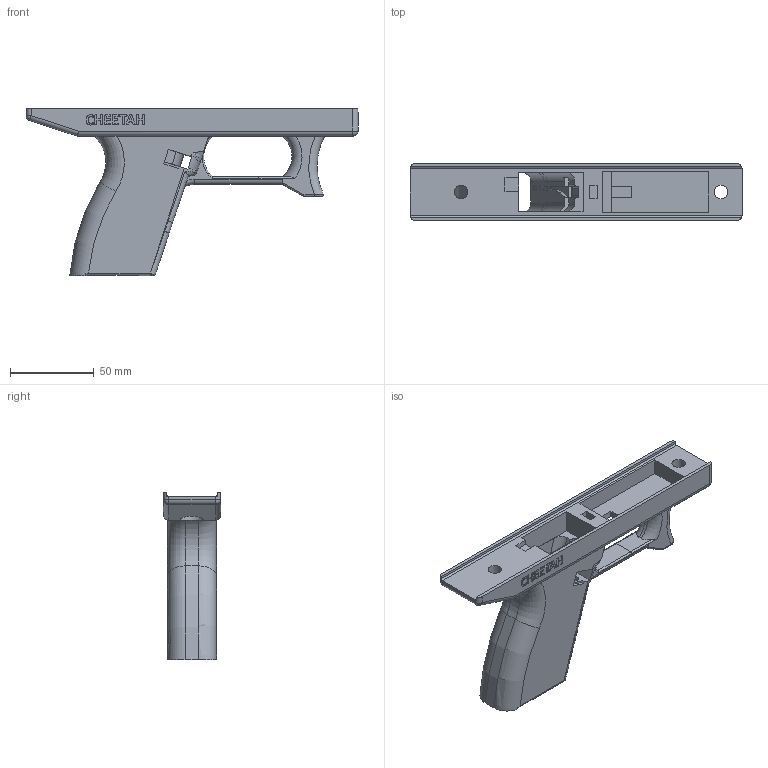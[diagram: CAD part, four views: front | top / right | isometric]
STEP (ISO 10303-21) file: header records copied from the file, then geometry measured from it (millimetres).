
FILE_DESCRIPTION(/* description */ (''),/* implementation_level */ '2;1');
FILE_NAME(/* name */ '',/* time_stamp */ '',/* author */ (''),/* organization */ (''),/* preprocessor_version */ 'ST-DEVELOPER v18.1',/* originating_system */ 'Autodesk Translation Framework v9.7.1.1290',/* authorisation */ '');
FILE_SCHEMA (('AUTOMOTIVE_DESIGN { 1 0 10303 214 3 1 1 }'));
Length unit declared in the file: millimetre
Products named in the file (1): Lower Receiver Body
Bounding box: 198 x 34 x 99.64 mm (x, y, z)
Volume: 126286.1 mm3; surface area: 50948.4 mm2
Topology: 1 solids, 2 shells, 562 faces, 1615 edges, 1061 vertices
Faces by surface type: bspline 256, plane 197, cylinder 82, torus 21, sphere 4, cone 2
Full cylindrical faces by diameter (mm): 1.3 x1, 7.973 x1, 8 x1, 14 x2
Entity records: 21927 total; most frequent: CARTESIAN_POINT 8839, ORIENTED_EDGE 3226, DIRECTION 1884, EDGE_CURVE 1613, VERTEX_POINT 1061, LINE 838, VECTOR 838, EDGE_LOOP 584
